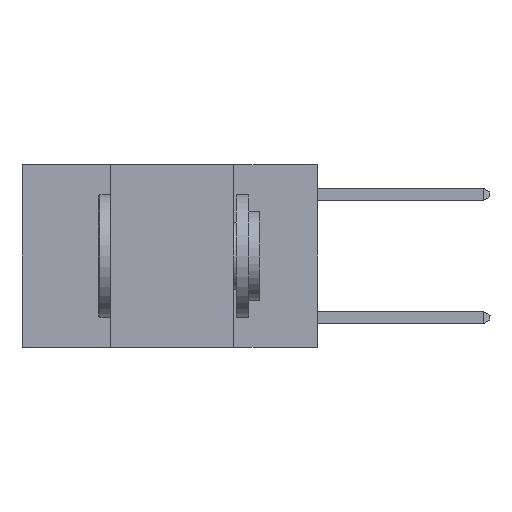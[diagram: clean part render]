
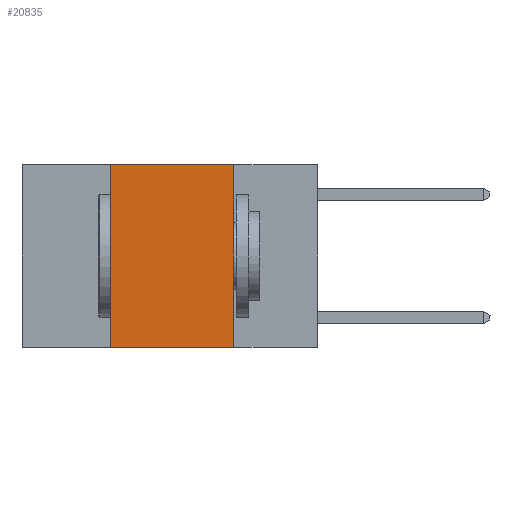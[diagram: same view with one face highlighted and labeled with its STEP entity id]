
A CAD part, left-side view. The second image highlights one B-rep face of the part: STEP entity #20835.
In plain terms, the highlighted planar face has unit normal (-1, 0, 0).
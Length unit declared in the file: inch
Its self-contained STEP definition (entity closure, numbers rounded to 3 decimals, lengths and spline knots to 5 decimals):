
#1027 = VERTEX_POINT ( 'NONE', #17707 ) ;
#2603 = PLANE ( 'NONE',  #27476 ) ;
#2907 = CARTESIAN_POINT ( 'NONE',  ( 0., 0.42, -0.37 ) ) ;
#3008 = VECTOR ( 'NONE', #5698, 39.37008 ) ;
#3338 = CARTESIAN_POINT ( 'NONE',  ( 0., 0.17, 0. ) ) ;
#4528 = VECTOR ( 'NONE', #21456, 39.37008 ) ;
#4865 = DIRECTION ( 'NONE',  ( 1., 0., 0. ) ) ;
#5698 = DIRECTION ( 'NONE',  ( 0., 0., -1. ) ) ;
#7363 = EDGE_CURVE ( 'NONE', #1027, #16149, #9015, .T. ) ;
#8090 = CARTESIAN_POINT ( 'NONE',  ( 0., 0.17, -0.37 ) ) ;
#9015 = LINE ( 'NONE', #3338, #3008 ) ;
#10630 = CARTESIAN_POINT ( 'NONE',  ( 0., 0.6, 0. ) ) ;
#10730 = ORIENTED_EDGE ( 'NONE', *, *, #16043, .F. ) ;
#13115 = EDGE_CURVE ( 'NONE', #28204, #1027, #23034, .T. ) ;
#15126 = CARTESIAN_POINT ( 'NONE',  ( 0., 0.6, -0.37 ) ) ;
#15195 = CARTESIAN_POINT ( 'NONE',  ( 0., 0.42, 0. ) ) ;
#16043 = EDGE_CURVE ( 'NONE', #17194, #28204, #23589, .T. ) ;
#16149 = VERTEX_POINT ( 'NONE', #8090 ) ;
#16174 = EDGE_CURVE ( 'NONE', #17194, #16149, #25301, .T. ) ;
#17194 = VERTEX_POINT ( 'NONE', #2907 ) ;
#17707 = CARTESIAN_POINT ( 'NONE',  ( 0., 0.17, 0. ) ) ;
#18722 = CARTESIAN_POINT ( 'NONE',  ( 0., 0.6, 0. ) ) ;
#19187 = CARTESIAN_POINT ( 'NONE',  ( 0., 0.42, 0. ) ) ;
#20052 = VECTOR ( 'NONE', #28452, 39.37008 ) ;
#20835 = ADVANCED_FACE ( 'NONE', ( #22131 ), #2603, .F. ) ;
#21004 = DIRECTION ( 'NONE',  ( 0., 0., -1. ) ) ;
#21456 = DIRECTION ( 'NONE',  ( 0., 0., 1. ) ) ;
#21607 = VECTOR ( 'NONE', #28719, 39.37008 ) ;
#21945 = EDGE_LOOP ( 'NONE', ( #28122, #28766, #10730, #28763 ) ) ;
#22131 = FACE_OUTER_BOUND ( 'NONE', #21945, .T. ) ;
#23034 = LINE ( 'NONE', #10630, #21607 ) ;
#23589 = LINE ( 'NONE', #19187, #4528 ) ;
#25301 = LINE ( 'NONE', #15126, #20052 ) ;
#27476 = AXIS2_PLACEMENT_3D ( 'NONE', #18722, #4865, #21004 ) ;
#28122 = ORIENTED_EDGE ( 'NONE', *, *, #7363, .F. ) ;
#28204 = VERTEX_POINT ( 'NONE', #15195 ) ;
#28452 = DIRECTION ( 'NONE',  ( 0., -1., 0. ) ) ;
#28719 = DIRECTION ( 'NONE',  ( 0., -1., 0. ) ) ;
#28763 = ORIENTED_EDGE ( 'NONE', *, *, #16174, .T. ) ;
#28766 = ORIENTED_EDGE ( 'NONE', *, *, #13115, .F. ) ;
